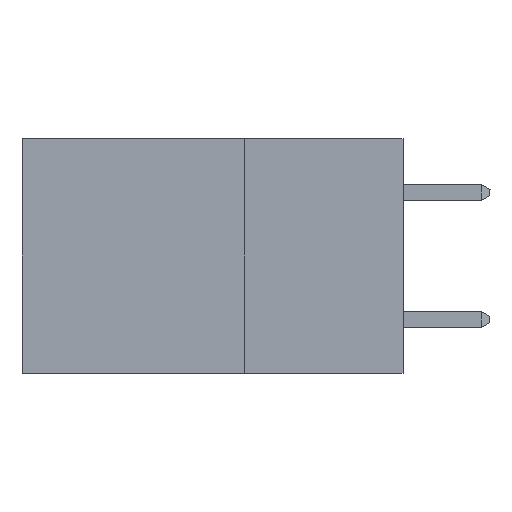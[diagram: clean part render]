
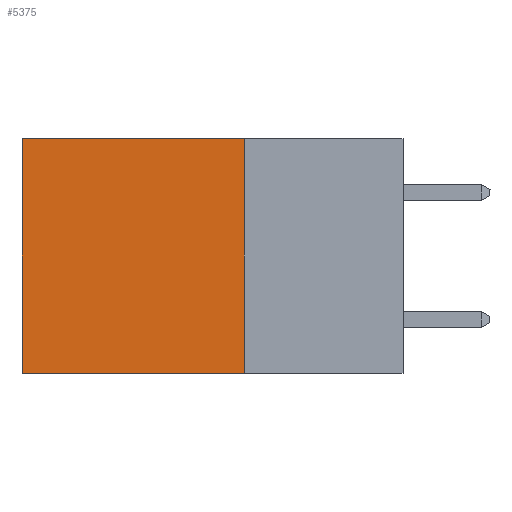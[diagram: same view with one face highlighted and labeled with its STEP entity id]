
A CAD part, left-side view. The second image highlights one B-rep face of the part: STEP entity #5375.
In plain terms, the highlighted planar face has unit normal (-1, 0, 0).
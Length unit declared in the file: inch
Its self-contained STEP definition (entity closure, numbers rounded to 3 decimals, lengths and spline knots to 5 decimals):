
#423 = CARTESIAN_POINT ( 'NONE',  ( 0.2875, 0.25, 0. ) ) ;
#484 = DIRECTION ( 'NONE',  ( 0., 0., -1. ) ) ;
#1064 = EDGE_CURVE ( 'NONE', #9317, #8612, #12692, .T. ) ;
#2081 = CARTESIAN_POINT ( 'NONE',  ( 0.2875, 0.25, 0. ) ) ;
#3012 = DIRECTION ( 'NONE',  ( 0., 0., -1. ) ) ;
#3134 = AXIS2_PLACEMENT_3D ( 'NONE', #10358, #12004, #3012 ) ;
#5373 = EDGE_CURVE ( 'NONE', #9924, #9317, #7749, .T. ) ;
#5375 = ADVANCED_FACE ( 'NONE', ( #13282 ), #14666, .F. ) ;
#5880 = EDGE_LOOP ( 'NONE', ( #7427, #14575, #10270, #14003 ) ) ;
#7427 = ORIENTED_EDGE ( 'NONE', *, *, #1064, .T. ) ;
#7749 = LINE ( 'NONE', #12496, #13625 ) ;
#8108 = EDGE_CURVE ( 'NONE', #12527, #8612, #13032, .T. ) ;
#8485 = CARTESIAN_POINT ( 'NONE',  ( 0.2875, 0.6, 0. ) ) ;
#8603 = DIRECTION ( 'NONE',  ( 0., 0., -1. ) ) ;
#8612 = VERTEX_POINT ( 'NONE', #12852 ) ;
#8786 = VECTOR ( 'NONE', #8603, 39.37008 ) ;
#9020 = DIRECTION ( 'NONE',  ( 0., 1., 0. ) ) ;
#9317 = VERTEX_POINT ( 'NONE', #8485 ) ;
#9750 = VECTOR ( 'NONE', #484, 39.37008 ) ;
#9924 = VERTEX_POINT ( 'NONE', #2081 ) ;
#10270 = ORIENTED_EDGE ( 'NONE', *, *, #10919, .F. ) ;
#10358 = CARTESIAN_POINT ( 'NONE',  ( 0.2875, 0.25, 0. ) ) ;
#10919 = EDGE_CURVE ( 'NONE', #9924, #12527, #11384, .T. ) ;
#11384 = LINE ( 'NONE', #423, #8786 ) ;
#11474 = CARTESIAN_POINT ( 'NONE',  ( 0.2875, 0.25, -0.37 ) ) ;
#12004 = DIRECTION ( 'NONE',  ( 1., 0., 0. ) ) ;
#12343 = VECTOR ( 'NONE', #14019, 39.37008 ) ;
#12496 = CARTESIAN_POINT ( 'NONE',  ( 0.2875, 0.25, 0. ) ) ;
#12527 = VERTEX_POINT ( 'NONE', #11474 ) ;
#12692 = LINE ( 'NONE', #13278, #9750 ) ;
#12852 = CARTESIAN_POINT ( 'NONE',  ( 0.2875, 0.6, -0.37 ) ) ;
#12917 = CARTESIAN_POINT ( 'NONE',  ( 0.2875, 0.25, -0.37 ) ) ;
#13032 = LINE ( 'NONE', #12917, #12343 ) ;
#13278 = CARTESIAN_POINT ( 'NONE',  ( 0.2875, 0.6, 0. ) ) ;
#13282 = FACE_OUTER_BOUND ( 'NONE', #5880, .T. ) ;
#13625 = VECTOR ( 'NONE', #9020, 39.37008 ) ;
#14003 = ORIENTED_EDGE ( 'NONE', *, *, #5373, .T. ) ;
#14019 = DIRECTION ( 'NONE',  ( 0., 1., 0. ) ) ;
#14575 = ORIENTED_EDGE ( 'NONE', *, *, #8108, .F. ) ;
#14666 = PLANE ( 'NONE',  #3134 ) ;
